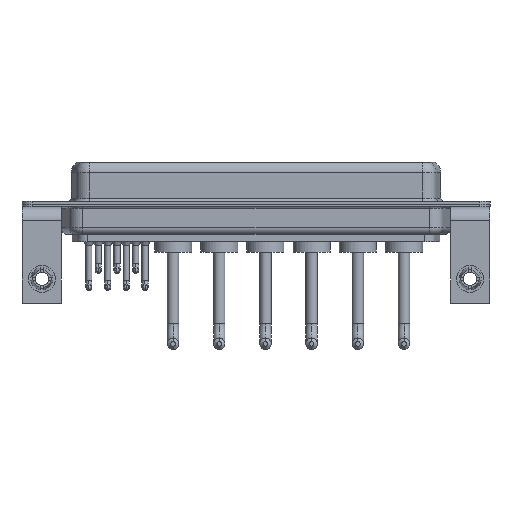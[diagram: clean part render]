
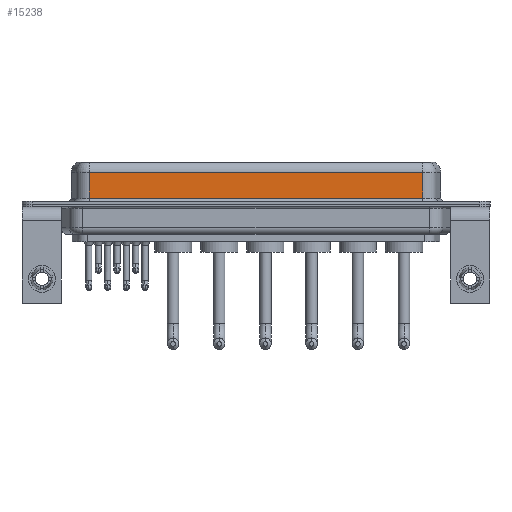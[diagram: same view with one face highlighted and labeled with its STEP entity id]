
A CAD part, front view. The second image highlights one B-rep face of the part: STEP entity #15238.
In plain terms, the highlighted planar face has unit normal (0, -1, 0).
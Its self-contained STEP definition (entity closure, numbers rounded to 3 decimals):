
#957 = CARTESIAN_POINT ( 'NONE',  ( 56.462, -3.95, 4.65 ) ) ;
#1140 = CARTESIAN_POINT ( 'NONE',  ( 7.038, -3.95, 4.65 ) ) ;
#1152 = DIRECTION ( 'NONE',  ( 0., 0., -1. ) ) ;
#1409 = EDGE_CURVE ( 'NONE', #14634, #20506, #14624, .T. ) ;
#3480 = FACE_OUTER_BOUND ( 'NONE', #9896, .T. ) ;
#4540 = VECTOR ( 'NONE', #1152, 1000. ) ;
#4860 = DIRECTION ( 'NONE',  ( 0., 0., 1. ) ) ;
#5683 = LINE ( 'NONE', #957, #7399 ) ;
#5982 = EDGE_CURVE ( 'NONE', #9142, #14634, #6081, .T. ) ;
#6081 = LINE ( 'NONE', #15759, #4540 ) ;
#7104 = CARTESIAN_POINT ( 'NONE',  ( 56.462, -3.95, 0.9 ) ) ;
#7399 = VECTOR ( 'NONE', #20224, 1000. ) ;
#7678 = AXIS2_PLACEMENT_3D ( 'NONE', #19685, #12844, #4860 ) ;
#8889 = DIRECTION ( 'NONE',  ( 1., 0., 0. ) ) ;
#9142 = VERTEX_POINT ( 'NONE', #1140 ) ;
#9389 = LINE ( 'NONE', #15820, #18094 ) ;
#9685 = ORIENTED_EDGE ( 'NONE', *, *, #14572, .F. ) ;
#9896 = EDGE_LOOP ( 'NONE', ( #9685, #17645, #10206, #15735 ) ) ;
#10206 = ORIENTED_EDGE ( 'NONE', *, *, #5982, .T. ) ;
#11590 = PLANE ( 'NONE',  #7678 ) ;
#11604 = CARTESIAN_POINT ( 'NONE',  ( 56.462, -3.95, 4.65 ) ) ;
#12049 = VECTOR ( 'NONE', #8889, 1000. ) ;
#12398 = VERTEX_POINT ( 'NONE', #11604 ) ;
#12735 = EDGE_CURVE ( 'NONE', #12398, #9142, #5683, .T. ) ;
#12844 = DIRECTION ( 'NONE',  ( 0., 1., 0. ) ) ;
#13830 = CARTESIAN_POINT ( 'NONE',  ( 56.462, -3.95, 0.9 ) ) ;
#14555 = CARTESIAN_POINT ( 'NONE',  ( 7.038, -3.95, 0.9 ) ) ;
#14572 = EDGE_CURVE ( 'NONE', #12398, #20506, #9389, .T. ) ;
#14624 = LINE ( 'NONE', #7104, #12049 ) ;
#14634 = VERTEX_POINT ( 'NONE', #14555 ) ;
#15238 = ADVANCED_FACE ( 'NONE', ( #3480 ), #11590, .F. ) ;
#15735 = ORIENTED_EDGE ( 'NONE', *, *, #1409, .T. ) ;
#15759 = CARTESIAN_POINT ( 'NONE',  ( 7.038, -3.95, 6.4 ) ) ;
#15820 = CARTESIAN_POINT ( 'NONE',  ( 56.462, -3.95, 6.4 ) ) ;
#17645 = ORIENTED_EDGE ( 'NONE', *, *, #12735, .T. ) ;
#18094 = VECTOR ( 'NONE', #19195, 1000. ) ;
#19195 = DIRECTION ( 'NONE',  ( 0., 0., -1. ) ) ;
#19685 = CARTESIAN_POINT ( 'NONE',  ( 56.462, -3.95, 6.4 ) ) ;
#20224 = DIRECTION ( 'NONE',  ( -1., 0., 0. ) ) ;
#20506 = VERTEX_POINT ( 'NONE', #13830 ) ;
